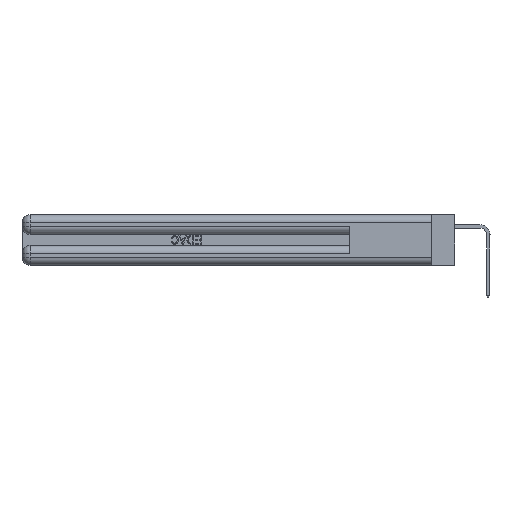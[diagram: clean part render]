
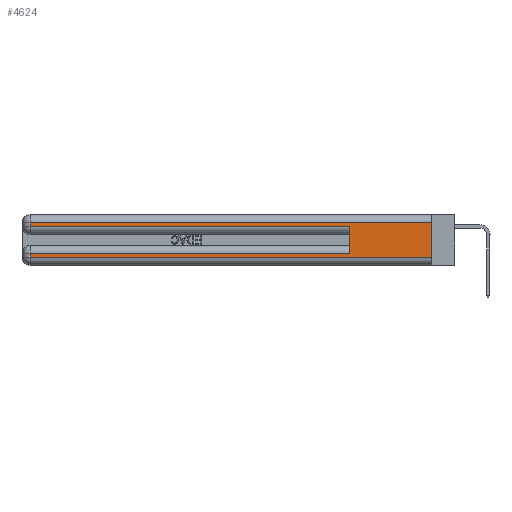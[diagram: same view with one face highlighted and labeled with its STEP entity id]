
A CAD part, left-side view. The second image highlights one B-rep face of the part: STEP entity #4624.
In plain terms, the highlighted planar face has unit normal (-1, 0, 0).
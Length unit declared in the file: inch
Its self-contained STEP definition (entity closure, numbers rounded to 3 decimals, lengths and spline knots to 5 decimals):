
#2539 = EDGE_CURVE ( 'NONE', #47904, #36102, #25882, .T. ) ;
#2547 = CARTESIAN_POINT ( 'NONE',  ( 0., 2.94, 0.37 ) ) ;
#3851 = CARTESIAN_POINT ( 'NONE',  ( 0., 0.6, 0.145 ) ) ;
#4296 = CARTESIAN_POINT ( 'NONE',  ( 0., 0., 0.285 ) ) ;
#4624 = ADVANCED_FACE ( 'NONE', ( #29340 ), #13595, .F. ) ;
#5152 = EDGE_CURVE ( 'NONE', #47904, #24319, #46156, .T. ) ;
#5164 = VECTOR ( 'NONE', #27161, 39.37008 ) ;
#5392 = VECTOR ( 'NONE', #10010, 39.37008 ) ;
#6125 = CARTESIAN_POINT ( 'NONE',  ( 0., 0., 0.31 ) ) ;
#7445 = VECTOR ( 'NONE', #46773, 39.37008 ) ;
#7920 = CARTESIAN_POINT ( 'NONE',  ( 0., 0., 0.06 ) ) ;
#8665 = LINE ( 'NONE', #27561, #7445 ) ;
#8888 = CARTESIAN_POINT ( 'NONE',  ( 0., 2.94, 0.06 ) ) ;
#10010 = DIRECTION ( 'NONE',  ( 0., 1., 0. ) ) ;
#10771 = LINE ( 'NONE', #2547, #49337 ) ;
#10960 = CARTESIAN_POINT ( 'NONE',  ( 0., 0., 0.06 ) ) ;
#11494 = VERTEX_POINT ( 'NONE', #46220 ) ;
#12431 = EDGE_LOOP ( 'NONE', ( #34492, #38116, #42944, #43555, #36967, #35163, #49002, #29183 ) ) ;
#12854 = CARTESIAN_POINT ( 'NONE',  ( 0., 2.94, 0.31 ) ) ;
#13595 = PLANE ( 'NONE',  #46616 ) ;
#14347 = LINE ( 'NONE', #7920, #43925 ) ;
#14787 = EDGE_CURVE ( 'NONE', #22466, #40987, #8665, .T. ) ;
#15032 = LINE ( 'NONE', #27024, #44623 ) ;
#16610 = VECTOR ( 'NONE', #23540, 39.37008 ) ;
#17404 = EDGE_CURVE ( 'NONE', #40987, #25442, #10771, .T. ) ;
#17484 = DIRECTION ( 'NONE',  ( 1., 0., 0. ) ) ;
#18069 = DIRECTION ( 'NONE',  ( 0., 0., -1. ) ) ;
#19687 = CARTESIAN_POINT ( 'NONE',  ( 0., 0., 0.31 ) ) ;
#19860 = CARTESIAN_POINT ( 'NONE',  ( 0., 2.94, 0.085 ) ) ;
#21589 = EDGE_CURVE ( 'NONE', #22466, #11494, #47404, .T. ) ;
#22466 = VERTEX_POINT ( 'NONE', #48859 ) ;
#23540 = DIRECTION ( 'NONE',  ( 0., -1., 0. ) ) ;
#24319 = VERTEX_POINT ( 'NONE', #10960 ) ;
#24664 = CARTESIAN_POINT ( 'NONE',  ( 0., 0., 0.37 ) ) ;
#25442 = VERTEX_POINT ( 'NONE', #8888 ) ;
#25882 = LINE ( 'NONE', #6125, #5392 ) ;
#27024 = CARTESIAN_POINT ( 'NONE',  ( 0., 2.94, 0.37 ) ) ;
#27161 = DIRECTION ( 'NONE',  ( 0., 0., 1. ) ) ;
#27561 = CARTESIAN_POINT ( 'NONE',  ( 0., 0., 0.085 ) ) ;
#28101 = LINE ( 'NONE', #4296, #16610 ) ;
#28595 = DIRECTION ( 'NONE',  ( 0., 0., -1. ) ) ;
#29183 = ORIENTED_EDGE ( 'NONE', *, *, #46821, .T. ) ;
#29340 = FACE_OUTER_BOUND ( 'NONE', #12431, .T. ) ;
#30899 = DIRECTION ( 'NONE',  ( 0., 0., -1. ) ) ;
#34492 = ORIENTED_EDGE ( 'NONE', *, *, #5152, .F. ) ;
#34576 = EDGE_CURVE ( 'NONE', #36102, #48287, #15032, .T. ) ;
#34693 = VECTOR ( 'NONE', #28595, 39.37008 ) ;
#35163 = ORIENTED_EDGE ( 'NONE', *, *, #14787, .T. ) ;
#36102 = VERTEX_POINT ( 'NONE', #12854 ) ;
#36967 = ORIENTED_EDGE ( 'NONE', *, *, #21589, .F. ) ;
#38116 = ORIENTED_EDGE ( 'NONE', *, *, #2539, .T. ) ;
#40605 = CARTESIAN_POINT ( 'NONE',  ( 0., 0., 0.37 ) ) ;
#40987 = VERTEX_POINT ( 'NONE', #19860 ) ;
#42944 = ORIENTED_EDGE ( 'NONE', *, *, #34576, .T. ) ;
#43555 = ORIENTED_EDGE ( 'NONE', *, *, #48413, .T. ) ;
#43925 = VECTOR ( 'NONE', #46511, 39.37008 ) ;
#44461 = DIRECTION ( 'NONE',  ( 0., 0., -1. ) ) ;
#44623 = VECTOR ( 'NONE', #30899, 39.37008 ) ;
#46156 = LINE ( 'NONE', #24664, #34693 ) ;
#46220 = CARTESIAN_POINT ( 'NONE',  ( 0., 0.6, 0.285 ) ) ;
#46511 = DIRECTION ( 'NONE',  ( 0., -1., 0. ) ) ;
#46616 = AXIS2_PLACEMENT_3D ( 'NONE', #40605, #17484, #44461 ) ;
#46773 = DIRECTION ( 'NONE',  ( 0., 1., 0. ) ) ;
#46821 = EDGE_CURVE ( 'NONE', #25442, #24319, #14347, .T. ) ;
#47404 = LINE ( 'NONE', #3851, #5164 ) ;
#47904 = VERTEX_POINT ( 'NONE', #19687 ) ;
#48287 = VERTEX_POINT ( 'NONE', #49664 ) ;
#48413 = EDGE_CURVE ( 'NONE', #48287, #11494, #28101, .T. ) ;
#48859 = CARTESIAN_POINT ( 'NONE',  ( 0., 0.6, 0.085 ) ) ;
#49002 = ORIENTED_EDGE ( 'NONE', *, *, #17404, .T. ) ;
#49337 = VECTOR ( 'NONE', #18069, 39.37008 ) ;
#49664 = CARTESIAN_POINT ( 'NONE',  ( 0., 2.94, 0.285 ) ) ;
